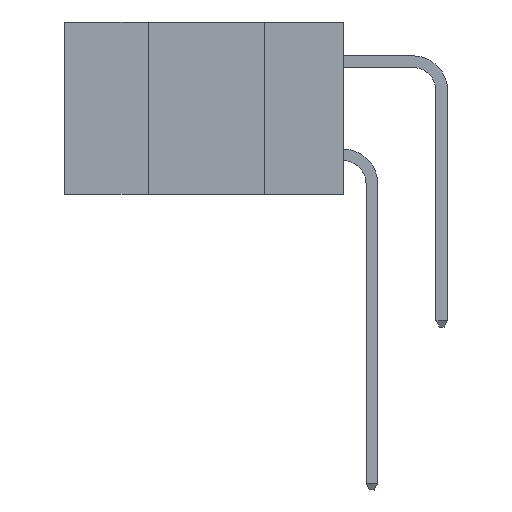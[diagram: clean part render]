
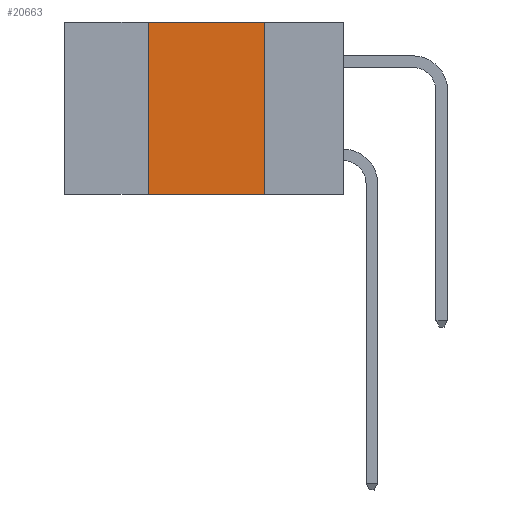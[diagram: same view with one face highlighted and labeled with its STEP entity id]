
A CAD part, left-side view. The second image highlights one B-rep face of the part: STEP entity #20663.
In plain terms, the highlighted planar face has unit normal (-1, 0, 0).
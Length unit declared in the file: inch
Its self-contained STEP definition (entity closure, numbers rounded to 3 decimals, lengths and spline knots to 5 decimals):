
#1389 = CARTESIAN_POINT ( 'NONE',  ( 0., 0.17, 0. ) ) ;
#1757 = LINE ( 'NONE', #1389, #22022 ) ;
#2029 = VECTOR ( 'NONE', #24363, 39.37008 ) ;
#2176 = VECTOR ( 'NONE', #7983, 39.37008 ) ;
#2242 = CARTESIAN_POINT ( 'NONE',  ( 0., 0.6, -0.37 ) ) ;
#3713 = AXIS2_PLACEMENT_3D ( 'NONE', #8616, #6786, #20128 ) ;
#4876 = VERTEX_POINT ( 'NONE', #11076 ) ;
#5015 = CARTESIAN_POINT ( 'NONE',  ( 0., 0.17, 0. ) ) ;
#6786 = DIRECTION ( 'NONE',  ( 1., 0., 0. ) ) ;
#7691 = LINE ( 'NONE', #20599, #2029 ) ;
#7941 = EDGE_CURVE ( 'NONE', #22239, #14371, #1757, .T. ) ;
#7983 = DIRECTION ( 'NONE',  ( 0., -1., 0. ) ) ;
#8616 = CARTESIAN_POINT ( 'NONE',  ( 0., 0.6, 0. ) ) ;
#8659 = FACE_OUTER_BOUND ( 'NONE', #23484, .T. ) ;
#9201 = ORIENTED_EDGE ( 'NONE', *, *, #7941, .F. ) ;
#10378 = ORIENTED_EDGE ( 'NONE', *, *, #17351, .F. ) ;
#10948 = EDGE_CURVE ( 'NONE', #4876, #14371, #17967, .T. ) ;
#11076 = CARTESIAN_POINT ( 'NONE',  ( 0., 0.42, -0.37 ) ) ;
#11217 = EDGE_CURVE ( 'NONE', #21447, #22239, #16456, .T. ) ;
#12786 = ORIENTED_EDGE ( 'NONE', *, *, #10948, .T. ) ;
#14365 = CARTESIAN_POINT ( 'NONE',  ( 0., 0.6, 0. ) ) ;
#14371 = VERTEX_POINT ( 'NONE', #17232 ) ;
#14703 = DIRECTION ( 'NONE',  ( 0., 0., -1. ) ) ;
#16456 = LINE ( 'NONE', #14365, #22746 ) ;
#17232 = CARTESIAN_POINT ( 'NONE',  ( 0., 0.17, -0.37 ) ) ;
#17351 = EDGE_CURVE ( 'NONE', #4876, #21447, #7691, .T. ) ;
#17967 = LINE ( 'NONE', #2242, #2176 ) ;
#18199 = PLANE ( 'NONE',  #3713 ) ;
#18209 = DIRECTION ( 'NONE',  ( 0., -1., 0. ) ) ;
#19344 = ORIENTED_EDGE ( 'NONE', *, *, #11217, .F. ) ;
#20128 = DIRECTION ( 'NONE',  ( 0., 0., -1. ) ) ;
#20599 = CARTESIAN_POINT ( 'NONE',  ( 0., 0.42, 0. ) ) ;
#20663 = ADVANCED_FACE ( 'NONE', ( #8659 ), #18199, .F. ) ;
#21447 = VERTEX_POINT ( 'NONE', #23768 ) ;
#22022 = VECTOR ( 'NONE', #14703, 39.37008 ) ;
#22239 = VERTEX_POINT ( 'NONE', #5015 ) ;
#22746 = VECTOR ( 'NONE', #18209, 39.37008 ) ;
#23484 = EDGE_LOOP ( 'NONE', ( #9201, #19344, #10378, #12786 ) ) ;
#23768 = CARTESIAN_POINT ( 'NONE',  ( 0., 0.42, 0. ) ) ;
#24363 = DIRECTION ( 'NONE',  ( 0., 0., 1. ) ) ;
